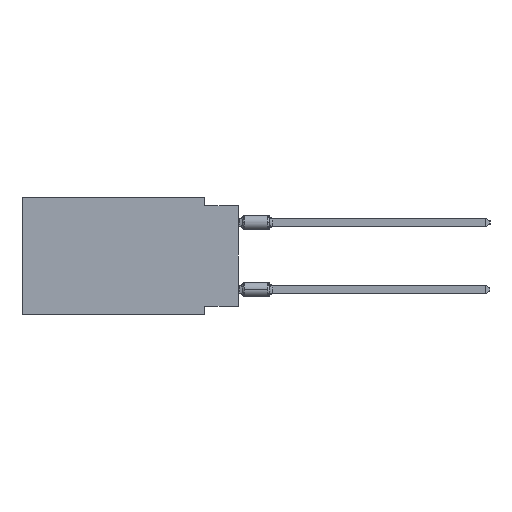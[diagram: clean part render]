
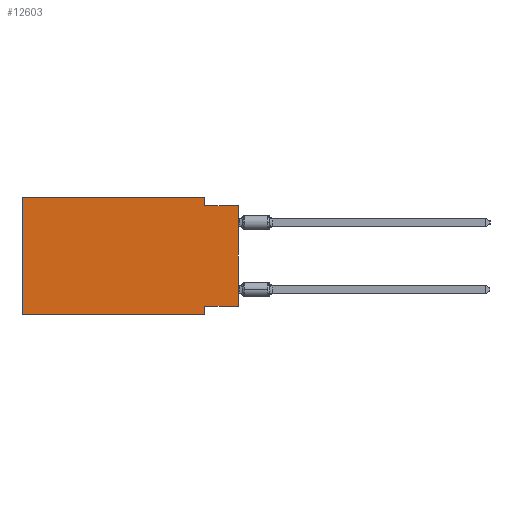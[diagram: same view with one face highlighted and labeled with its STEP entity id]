
A CAD part, left-side view. The second image highlights one B-rep face of the part: STEP entity #12603.
In plain terms, the highlighted planar face has unit normal (-1, 0, 0).
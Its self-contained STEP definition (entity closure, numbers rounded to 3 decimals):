
#279 = VERTEX_POINT ( 'NONE', #8568 ) ;
#280 = CARTESIAN_POINT ( 'NONE',  ( 0., 2.54, -8.255 ) ) ;
#689 = DIRECTION ( 'NONE',  ( 0., -1., 0. ) ) ;
#1104 = CARTESIAN_POINT ( 'NONE',  ( 0., 2.54, -0.635 ) ) ;
#1591 = LINE ( 'NONE', #19182, #22431 ) ;
#1920 = VECTOR ( 'NONE', #689, 1000. ) ;
#2137 = EDGE_CURVE ( 'NONE', #11071, #5877, #11404, .T. ) ;
#3070 = LINE ( 'NONE', #18710, #21119 ) ;
#3119 = CARTESIAN_POINT ( 'NONE',  ( 0., 0., 0. ) ) ;
#3558 = DIRECTION ( 'NONE',  ( 0., 0., 1. ) ) ;
#3717 = DIRECTION ( 'NONE',  ( 0., 1., 0. ) ) ;
#3973 = CARTESIAN_POINT ( 'NONE',  ( 0., 2.54, -8.89 ) ) ;
#5172 = DIRECTION ( 'NONE',  ( 0., -1., 0. ) ) ;
#5781 = LINE ( 'NONE', #17768, #11207 ) ;
#5877 = VERTEX_POINT ( 'NONE', #1104 ) ;
#5893 = CARTESIAN_POINT ( 'NONE',  ( 0., 0., -0.635 ) ) ;
#6590 = ORIENTED_EDGE ( 'NONE', *, *, #7158, .F. ) ;
#6682 = CARTESIAN_POINT ( 'NONE',  ( 0., 16.383, -8.89 ) ) ;
#6888 = EDGE_CURVE ( 'NONE', #279, #13519, #12195, .T. ) ;
#7158 = EDGE_CURVE ( 'NONE', #20661, #11071, #1591, .T. ) ;
#7724 = CARTESIAN_POINT ( 'NONE',  ( 0., 0., -0.635 ) ) ;
#8521 = ORIENTED_EDGE ( 'NONE', *, *, #15411, .F. ) ;
#8568 = CARTESIAN_POINT ( 'NONE',  ( 0., 16.383, -8.89 ) ) ;
#8784 = FACE_OUTER_BOUND ( 'NONE', #19833, .T. ) ;
#8957 = VECTOR ( 'NONE', #16248, 1000. ) ;
#9099 = ORIENTED_EDGE ( 'NONE', *, *, #14743, .T. ) ;
#10284 = DIRECTION ( 'NONE',  ( 0., 0., -1. ) ) ;
#10500 = VERTEX_POINT ( 'NONE', #16204 ) ;
#10876 = CARTESIAN_POINT ( 'NONE',  ( 0., 2.54, 0. ) ) ;
#11071 = VERTEX_POINT ( 'NONE', #10876 ) ;
#11207 = VECTOR ( 'NONE', #3717, 1000. ) ;
#11404 = LINE ( 'NONE', #13133, #8957 ) ;
#11498 = EDGE_CURVE ( 'NONE', #10500, #21653, #5781, .T. ) ;
#11687 = DIRECTION ( 'NONE',  ( 0., 0., 1. ) ) ;
#12195 = LINE ( 'NONE', #6682, #19461 ) ;
#12304 = DIRECTION ( 'NONE',  ( 0., 0., -1. ) ) ;
#12308 = LINE ( 'NONE', #3119, #21074 ) ;
#12352 = CARTESIAN_POINT ( 'NONE',  ( 0., 16.383, 0. ) ) ;
#12603 = ADVANCED_FACE ( 'NONE', ( #8784 ), #19266, .F. ) ;
#12735 = ORIENTED_EDGE ( 'NONE', *, *, #11498, .F. ) ;
#13017 = ORIENTED_EDGE ( 'NONE', *, *, #18683, .F. ) ;
#13091 = ORIENTED_EDGE ( 'NONE', *, *, #19091, .F. ) ;
#13133 = CARTESIAN_POINT ( 'NONE',  ( 0., 2.54, 0. ) ) ;
#13519 = VERTEX_POINT ( 'NONE', #19669 ) ;
#13746 = VECTOR ( 'NONE', #12304, 1000. ) ;
#14024 = LINE ( 'NONE', #3973, #13746 ) ;
#14743 = EDGE_CURVE ( 'NONE', #10500, #22310, #12308, .T. ) ;
#14867 = LINE ( 'NONE', #7724, #1920 ) ;
#15411 = EDGE_CURVE ( 'NONE', #5877, #22310, #14867, .T. ) ;
#16204 = CARTESIAN_POINT ( 'NONE',  ( 0., 0., -8.255 ) ) ;
#16222 = AXIS2_PLACEMENT_3D ( 'NONE', #12352, #17201, #10284 ) ;
#16248 = DIRECTION ( 'NONE',  ( 0., 0., -1. ) ) ;
#16970 = CARTESIAN_POINT ( 'NONE',  ( 0., 16.383, 0. ) ) ;
#17201 = DIRECTION ( 'NONE',  ( 1., 0., 0. ) ) ;
#17586 = ORIENTED_EDGE ( 'NONE', *, *, #2137, .F. ) ;
#17768 = CARTESIAN_POINT ( 'NONE',  ( 0., 0., -8.255 ) ) ;
#18683 = EDGE_CURVE ( 'NONE', #21653, #13519, #14024, .T. ) ;
#18710 = CARTESIAN_POINT ( 'NONE',  ( 0., 16.383, 0. ) ) ;
#19091 = EDGE_CURVE ( 'NONE', #279, #20661, #3070, .T. ) ;
#19182 = CARTESIAN_POINT ( 'NONE',  ( 0., 16.383, 0. ) ) ;
#19266 = PLANE ( 'NONE',  #16222 ) ;
#19461 = VECTOR ( 'NONE', #5172, 1000. ) ;
#19669 = CARTESIAN_POINT ( 'NONE',  ( 0., 2.54, -8.89 ) ) ;
#19833 = EDGE_LOOP ( 'NONE', ( #9099, #8521, #17586, #6590, #13091, #21788, #13017, #12735 ) ) ;
#20661 = VERTEX_POINT ( 'NONE', #16970 ) ;
#21074 = VECTOR ( 'NONE', #3558, 1000. ) ;
#21119 = VECTOR ( 'NONE', #11687, 1000. ) ;
#21259 = DIRECTION ( 'NONE',  ( 0., -1., 0. ) ) ;
#21653 = VERTEX_POINT ( 'NONE', #280 ) ;
#21788 = ORIENTED_EDGE ( 'NONE', *, *, #6888, .T. ) ;
#22310 = VERTEX_POINT ( 'NONE', #5893 ) ;
#22431 = VECTOR ( 'NONE', #21259, 1000. ) ;
